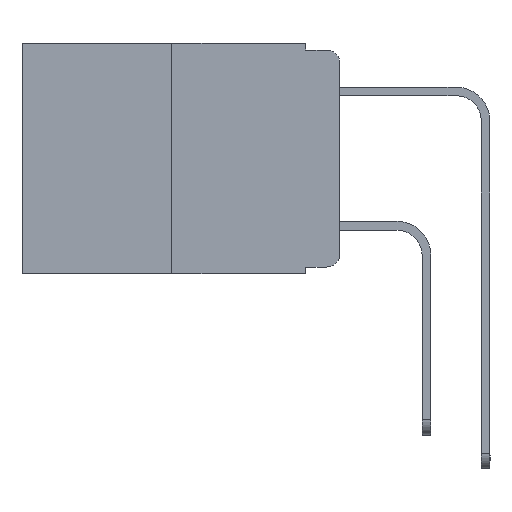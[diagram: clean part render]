
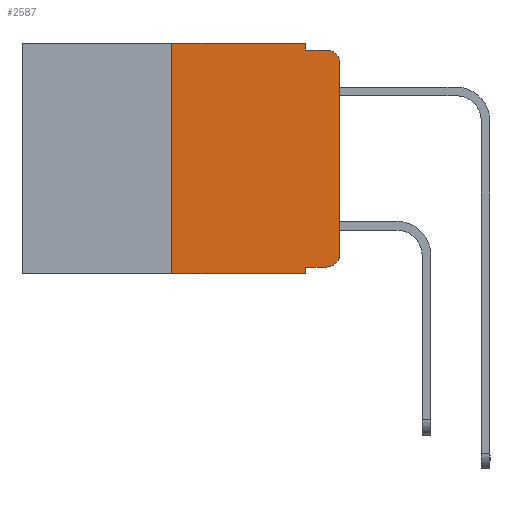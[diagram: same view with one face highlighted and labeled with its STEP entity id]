
A CAD part, left-side view. The second image highlights one B-rep face of the part: STEP entity #2587.
In plain terms, the highlighted planar face has unit normal (-1, 0, 0).
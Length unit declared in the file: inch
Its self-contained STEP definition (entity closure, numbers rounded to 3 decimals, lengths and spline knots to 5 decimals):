
#16 = CARTESIAN_POINT ( 'NONE',  ( 0., 0.25, -0.343 ) ) ;
#97 = ORIENTED_EDGE ( 'NONE', *, *, #6426, .F. ) ;
#147 = VERTEX_POINT ( 'NONE', #15656 ) ;
#498 = VECTOR ( 'NONE', #18738, 39.37008 ) ;
#642 = LINE ( 'NONE', #12151, #17221 ) ;
#669 = DIRECTION ( 'NONE',  ( -1., 0., 0. ) ) ;
#1064 = EDGE_CURVE ( 'NONE', #11953, #5100, #5934, .T. ) ;
#1387 = CARTESIAN_POINT ( 'NONE',  ( 0., 0.02, -0.313 ) ) ;
#1775 = VERTEX_POINT ( 'NONE', #16723 ) ;
#1957 = EDGE_CURVE ( 'NONE', #6631, #13722, #12019, .T. ) ;
#1976 = EDGE_CURVE ( 'NONE', #12981, #3447, #13769, .T. ) ;
#2100 = LINE ( 'NONE', #17432, #6463 ) ;
#2220 = DIRECTION ( 'NONE',  ( 0., -1., 0. ) ) ;
#2265 = DIRECTION ( 'NONE',  ( 0., 0., 1. ) ) ;
#2587 = ADVANCED_FACE ( 'NONE', ( #6288 ), #19075, .F. ) ;
#2612 = DIRECTION ( 'NONE',  ( -1., 0., 0. ) ) ;
#2955 = VERTEX_POINT ( 'NONE', #6571 ) ;
#2976 = ORIENTED_EDGE ( 'NONE', *, *, #17050, .T. ) ;
#2993 = ORIENTED_EDGE ( 'NONE', *, *, #1064, .T. ) ;
#3086 = VECTOR ( 'NONE', #19103, 39.37008 ) ;
#3279 = EDGE_CURVE ( 'NONE', #6631, #3447, #2100, .T. ) ;
#3447 = VERTEX_POINT ( 'NONE', #21348 ) ;
#3689 = CARTESIAN_POINT ( 'NONE',  ( 0., 0.25, 0. ) ) ;
#3976 = CARTESIAN_POINT ( 'NONE',  ( 0., 0.051, -0.333 ) ) ;
#4024 = DIRECTION ( 'NONE',  ( 0., 0., 1. ) ) ;
#4101 = CARTESIAN_POINT ( 'NONE',  ( 0., 0.473, 0. ) ) ;
#4423 = VECTOR ( 'NONE', #2220, 39.37008 ) ;
#4430 = VERTEX_POINT ( 'NONE', #12897 ) ;
#5012 = EDGE_CURVE ( 'NONE', #12981, #147, #15040, .T. ) ;
#5100 = VERTEX_POINT ( 'NONE', #5628 ) ;
#5482 = CARTESIAN_POINT ( 'NONE',  ( 0., 0.25, 0. ) ) ;
#5609 = EDGE_CURVE ( 'NONE', #147, #2955, #21418, .T. ) ;
#5628 = CARTESIAN_POINT ( 'NONE',  ( 0., 0.02, -0.01 ) ) ;
#5934 = CIRCLE ( 'NONE', #17115, 0.02 ) ;
#6288 = FACE_OUTER_BOUND ( 'NONE', #8306, .T. ) ;
#6426 = EDGE_CURVE ( 'NONE', #4430, #5100, #20714, .T. ) ;
#6463 = VECTOR ( 'NONE', #12191, 39.37008 ) ;
#6480 = ORIENTED_EDGE ( 'NONE', *, *, #14094, .F. ) ;
#6571 = CARTESIAN_POINT ( 'NONE',  ( 0., 0., -0.313 ) ) ;
#6631 = VERTEX_POINT ( 'NONE', #16 ) ;
#6980 = CARTESIAN_POINT ( 'NONE',  ( 0., 0.051, 0. ) ) ;
#7324 = DIRECTION ( 'NONE',  ( 0., -1., 0. ) ) ;
#8306 = EDGE_LOOP ( 'NONE', ( #2976, #2993, #97, #6480, #11341, #9774, #20946, #18181, #17777, #14228 ) ) ;
#9108 = DIRECTION ( 'NONE',  ( 0., 0., -1. ) ) ;
#9140 = DIRECTION ( 'NONE',  ( 1., 0., 0. ) ) ;
#9774 = ORIENTED_EDGE ( 'NONE', *, *, #1957, .F. ) ;
#10023 = CARTESIAN_POINT ( 'NONE',  ( 0., 0.051, 0. ) ) ;
#10340 = CARTESIAN_POINT ( 'NONE',  ( 0., 0.051, -0.333 ) ) ;
#11207 = CARTESIAN_POINT ( 'NONE',  ( 0., 0., -0.03 ) ) ;
#11341 = ORIENTED_EDGE ( 'NONE', *, *, #19470, .F. ) ;
#11779 = LINE ( 'NONE', #10023, #17189 ) ;
#11953 = VERTEX_POINT ( 'NONE', #11207 ) ;
#12019 = LINE ( 'NONE', #3689, #14295 ) ;
#12093 = CARTESIAN_POINT ( 'NONE',  ( 0., 0.051, -0.01 ) ) ;
#12151 = CARTESIAN_POINT ( 'NONE',  ( 0., 0.473, 0. ) ) ;
#12191 = DIRECTION ( 'NONE',  ( 0., -1., 0. ) ) ;
#12465 = CARTESIAN_POINT ( 'NONE',  ( 0., 0., 0. ) ) ;
#12897 = CARTESIAN_POINT ( 'NONE',  ( 0., 0.051, -0.01 ) ) ;
#12981 = VERTEX_POINT ( 'NONE', #10340 ) ;
#13062 = VECTOR ( 'NONE', #4024, 39.37008 ) ;
#13722 = VERTEX_POINT ( 'NONE', #5482 ) ;
#13769 = LINE ( 'NONE', #6980, #3086 ) ;
#14094 = EDGE_CURVE ( 'NONE', #1775, #4430, #11779, .T. ) ;
#14228 = ORIENTED_EDGE ( 'NONE', *, *, #5609, .T. ) ;
#14295 = VECTOR ( 'NONE', #2265, 39.37008 ) ;
#15040 = LINE ( 'NONE', #3976, #4423 ) ;
#15133 = AXIS2_PLACEMENT_3D ( 'NONE', #1387, #2612, #19325 ) ;
#15573 = AXIS2_PLACEMENT_3D ( 'NONE', #4101, #9140, #15819 ) ;
#15636 = LINE ( 'NONE', #12465, #13062 ) ;
#15656 = CARTESIAN_POINT ( 'NONE',  ( 0., 0.02, -0.333 ) ) ;
#15685 = CARTESIAN_POINT ( 'NONE',  ( 0., 0.02, -0.03 ) ) ;
#15819 = DIRECTION ( 'NONE',  ( 0., 0., -1. ) ) ;
#16723 = CARTESIAN_POINT ( 'NONE',  ( 0., 0.051, 0. ) ) ;
#17050 = EDGE_CURVE ( 'NONE', #2955, #11953, #15636, .T. ) ;
#17115 = AXIS2_PLACEMENT_3D ( 'NONE', #15685, #669, #9108 ) ;
#17189 = VECTOR ( 'NONE', #21609, 39.37008 ) ;
#17221 = VECTOR ( 'NONE', #7324, 39.37008 ) ;
#17432 = CARTESIAN_POINT ( 'NONE',  ( 0., 0.473, -0.343 ) ) ;
#17777 = ORIENTED_EDGE ( 'NONE', *, *, #5012, .T. ) ;
#18181 = ORIENTED_EDGE ( 'NONE', *, *, #1976, .F. ) ;
#18738 = DIRECTION ( 'NONE',  ( 0., -1., 0. ) ) ;
#19075 = PLANE ( 'NONE',  #15573 ) ;
#19103 = DIRECTION ( 'NONE',  ( 0., 0., -1. ) ) ;
#19325 = DIRECTION ( 'NONE',  ( 0., 0., -1. ) ) ;
#19470 = EDGE_CURVE ( 'NONE', #13722, #1775, #642, .T. ) ;
#20714 = LINE ( 'NONE', #12093, #498 ) ;
#20946 = ORIENTED_EDGE ( 'NONE', *, *, #3279, .T. ) ;
#21348 = CARTESIAN_POINT ( 'NONE',  ( 0., 0.051, -0.343 ) ) ;
#21418 = CIRCLE ( 'NONE', #15133, 0.02 ) ;
#21609 = DIRECTION ( 'NONE',  ( 0., 0., -1. ) ) ;
